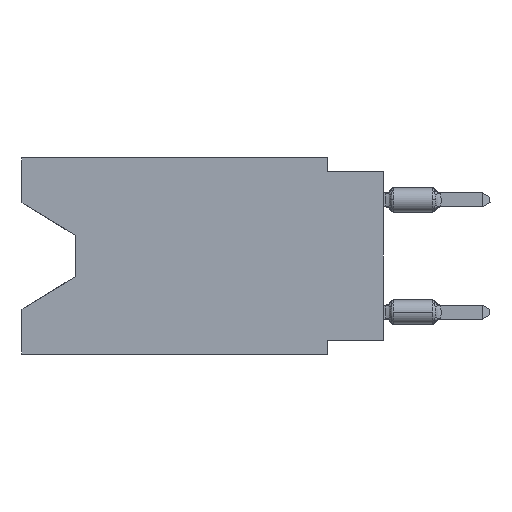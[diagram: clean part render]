
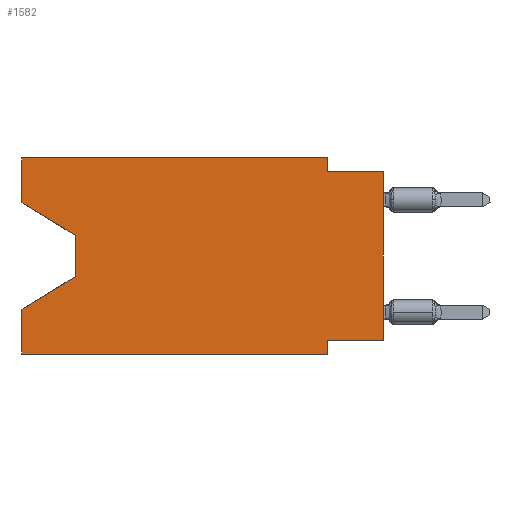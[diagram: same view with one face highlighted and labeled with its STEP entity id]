
A CAD part, left-side view. The second image highlights one B-rep face of the part: STEP entity #1582.
In plain terms, the highlighted planar face has unit normal (-1, 0, 0).
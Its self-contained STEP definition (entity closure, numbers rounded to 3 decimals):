
#602 = CARTESIAN_POINT ( 'NONE',  ( 0., 0., -0.635 ) ) ;
#934 = LINE ( 'NONE', #16400, #3394 ) ;
#997 = CARTESIAN_POINT ( 'NONE',  ( 0., 16.383, -2.038 ) ) ;
#1052 = VERTEX_POINT ( 'NONE', #17905 ) ;
#1582 = ADVANCED_FACE ( 'NONE', ( #11110 ), #7100, .F. ) ;
#2451 = ORIENTED_EDGE ( 'NONE', *, *, #4876, .F. ) ;
#2466 = VECTOR ( 'NONE', #6630, 1000. ) ;
#2510 = CARTESIAN_POINT ( 'NONE',  ( 0., 2.54, -8.255 ) ) ;
#2584 = CARTESIAN_POINT ( 'NONE',  ( 0., 2.54, 0. ) ) ;
#2668 = EDGE_CURVE ( 'NONE', #10058, #19296, #21754, .T. ) ;
#2710 = DIRECTION ( 'NONE',  ( 0., 0., -1. ) ) ;
#2850 = EDGE_LOOP ( 'NONE', ( #17248, #6917, #3178, #2451, #3767, #16743, #11755, #4930, #4862, #7714, #5657, #7864 ) ) ;
#2857 = VERTEX_POINT ( 'NONE', #23232 ) ;
#3060 = CARTESIAN_POINT ( 'NONE',  ( 0., 16.383, 0. ) ) ;
#3178 = ORIENTED_EDGE ( 'NONE', *, *, #8019, .T. ) ;
#3394 = VECTOR ( 'NONE', #12545, 1000. ) ;
#3433 = LINE ( 'NONE', #22417, #19672 ) ;
#3767 = ORIENTED_EDGE ( 'NONE', *, *, #7741, .T. ) ;
#4641 = CARTESIAN_POINT ( 'NONE',  ( 0., 2.54, -8.89 ) ) ;
#4646 = DIRECTION ( 'NONE',  ( 0., 0.855, -0.519 ) ) ;
#4862 = ORIENTED_EDGE ( 'NONE', *, *, #21485, .F. ) ;
#4868 = VERTEX_POINT ( 'NONE', #18177 ) ;
#4876 = EDGE_CURVE ( 'NONE', #13280, #6946, #11168, .T. ) ;
#4930 = ORIENTED_EDGE ( 'NONE', *, *, #6084, .T. ) ;
#5172 = CARTESIAN_POINT ( 'NONE',  ( 0., 13.97, -3.505 ) ) ;
#5437 = VERTEX_POINT ( 'NONE', #5985 ) ;
#5483 = DIRECTION ( 'NONE',  ( 0., 0., -1. ) ) ;
#5657 = ORIENTED_EDGE ( 'NONE', *, *, #21654, .F. ) ;
#5985 = CARTESIAN_POINT ( 'NONE',  ( 0., 2.54, -0.635 ) ) ;
#6017 = EDGE_CURVE ( 'NONE', #2857, #5437, #10452, .T. ) ;
#6084 = EDGE_CURVE ( 'NONE', #13479, #19345, #3433, .T. ) ;
#6181 = CARTESIAN_POINT ( 'NONE',  ( 0., 0., -8.255 ) ) ;
#6589 = LINE ( 'NONE', #20087, #15016 ) ;
#6630 = DIRECTION ( 'NONE',  ( 0., 0., -1. ) ) ;
#6721 = VECTOR ( 'NONE', #8230, 1000. ) ;
#6873 = VECTOR ( 'NONE', #2710, 1000. ) ;
#6917 = ORIENTED_EDGE ( 'NONE', *, *, #9229, .T. ) ;
#6946 = VERTEX_POINT ( 'NONE', #10743 ) ;
#7100 = PLANE ( 'NONE',  #12400 ) ;
#7391 = LINE ( 'NONE', #22152, #8871 ) ;
#7714 = ORIENTED_EDGE ( 'NONE', *, *, #6017, .F. ) ;
#7741 = EDGE_CURVE ( 'NONE', #13280, #19296, #7391, .T. ) ;
#7864 = ORIENTED_EDGE ( 'NONE', *, *, #9148, .F. ) ;
#8019 = EDGE_CURVE ( 'NONE', #4868, #6946, #15890, .T. ) ;
#8199 = DIRECTION ( 'NONE',  ( 0., -1., 0. ) ) ;
#8230 = DIRECTION ( 'NONE',  ( 0., -0.855, -0.519 ) ) ;
#8799 = DIRECTION ( 'NONE',  ( 0., 0., 1. ) ) ;
#8871 = VECTOR ( 'NONE', #12902, 1000. ) ;
#9148 = EDGE_CURVE ( 'NONE', #9343, #20597, #20180, .T. ) ;
#9161 = DIRECTION ( 'NONE',  ( 0., 0., -1. ) ) ;
#9229 = EDGE_CURVE ( 'NONE', #1052, #4868, #20918, .T. ) ;
#9343 = VERTEX_POINT ( 'NONE', #9665 ) ;
#9665 = CARTESIAN_POINT ( 'NONE',  ( 0., 16.383, -2.038 ) ) ;
#10003 = CARTESIAN_POINT ( 'NONE',  ( 0., 0., -0.635 ) ) ;
#10058 = VERTEX_POINT ( 'NONE', #2510 ) ;
#10452 = LINE ( 'NONE', #2584, #6873 ) ;
#10678 = DIRECTION ( 'NONE',  ( 0., 0., 1. ) ) ;
#10743 = CARTESIAN_POINT ( 'NONE',  ( 0., 16.383, -6.852 ) ) ;
#11110 = FACE_OUTER_BOUND ( 'NONE', #2850, .T. ) ;
#11168 = LINE ( 'NONE', #14545, #13223 ) ;
#11439 = CARTESIAN_POINT ( 'NONE',  ( 0., 16.383, -8.89 ) ) ;
#11755 = ORIENTED_EDGE ( 'NONE', *, *, #17532, .F. ) ;
#12400 = AXIS2_PLACEMENT_3D ( 'NONE', #16850, #24221, #5483 ) ;
#12545 = DIRECTION ( 'NONE',  ( 0., 1., 0. ) ) ;
#12902 = DIRECTION ( 'NONE',  ( 0., -1., 0. ) ) ;
#13223 = VECTOR ( 'NONE', #16789, 1000. ) ;
#13280 = VERTEX_POINT ( 'NONE', #11439 ) ;
#13479 = VERTEX_POINT ( 'NONE', #6181 ) ;
#14545 = CARTESIAN_POINT ( 'NONE',  ( 0., 16.383, 0. ) ) ;
#14582 = EDGE_CURVE ( 'NONE', #9343, #1052, #18110, .T. ) ;
#15016 = VECTOR ( 'NONE', #19966, 1000. ) ;
#15890 = LINE ( 'NONE', #19641, #21666 ) ;
#16400 = CARTESIAN_POINT ( 'NONE',  ( 0., 0., -8.255 ) ) ;
#16599 = VECTOR ( 'NONE', #8199, 1000. ) ;
#16743 = ORIENTED_EDGE ( 'NONE', *, *, #2668, .F. ) ;
#16789 = DIRECTION ( 'NONE',  ( 0., 0., 1. ) ) ;
#16850 = CARTESIAN_POINT ( 'NONE',  ( 0., 16.383, 0. ) ) ;
#17248 = ORIENTED_EDGE ( 'NONE', *, *, #14582, .T. ) ;
#17532 = EDGE_CURVE ( 'NONE', #13479, #10058, #934, .T. ) ;
#17649 = CARTESIAN_POINT ( 'NONE',  ( 0., 16.383, 0. ) ) ;
#17905 = CARTESIAN_POINT ( 'NONE',  ( 0., 13.97, -3.505 ) ) ;
#18110 = LINE ( 'NONE', #997, #6721 ) ;
#18177 = CARTESIAN_POINT ( 'NONE',  ( 0., 13.97, -5.385 ) ) ;
#19296 = VERTEX_POINT ( 'NONE', #20881 ) ;
#19345 = VERTEX_POINT ( 'NONE', #10003 ) ;
#19346 = LINE ( 'NONE', #602, #16599 ) ;
#19641 = CARTESIAN_POINT ( 'NONE',  ( 0., 13.97, -5.385 ) ) ;
#19672 = VECTOR ( 'NONE', #8799, 1000. ) ;
#19966 = DIRECTION ( 'NONE',  ( 0., -1., 0. ) ) ;
#20087 = CARTESIAN_POINT ( 'NONE',  ( 0., 16.383, 0. ) ) ;
#20180 = LINE ( 'NONE', #3060, #22313 ) ;
#20597 = VERTEX_POINT ( 'NONE', #17649 ) ;
#20881 = CARTESIAN_POINT ( 'NONE',  ( 0., 2.54, -8.89 ) ) ;
#20918 = LINE ( 'NONE', #5172, #23539 ) ;
#21485 = EDGE_CURVE ( 'NONE', #5437, #19345, #19346, .T. ) ;
#21654 = EDGE_CURVE ( 'NONE', #20597, #2857, #6589, .T. ) ;
#21666 = VECTOR ( 'NONE', #4646, 1000. ) ;
#21754 = LINE ( 'NONE', #4641, #2466 ) ;
#22152 = CARTESIAN_POINT ( 'NONE',  ( 0., 16.383, -8.89 ) ) ;
#22313 = VECTOR ( 'NONE', #10678, 1000. ) ;
#22417 = CARTESIAN_POINT ( 'NONE',  ( 0., 0., 0. ) ) ;
#23232 = CARTESIAN_POINT ( 'NONE',  ( 0., 2.54, 0. ) ) ;
#23539 = VECTOR ( 'NONE', #9161, 1000. ) ;
#24221 = DIRECTION ( 'NONE',  ( 1., 0., 0. ) ) ;
